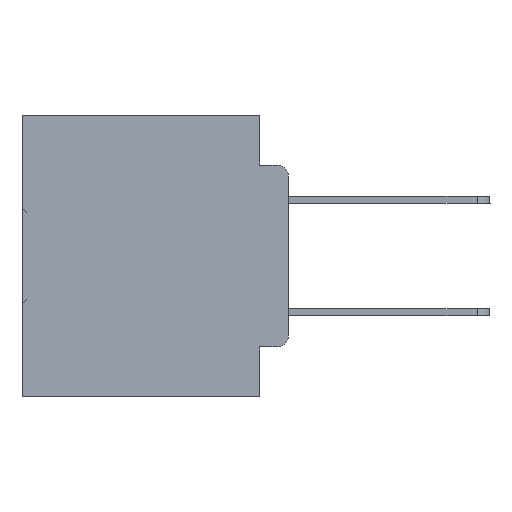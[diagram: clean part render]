
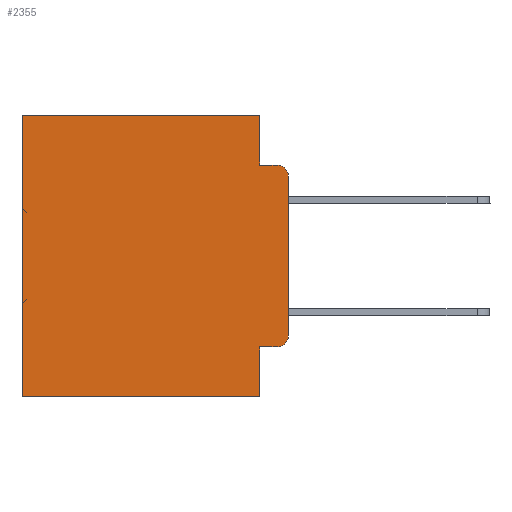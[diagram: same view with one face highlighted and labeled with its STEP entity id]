
A CAD part, left-side view. The second image highlights one B-rep face of the part: STEP entity #2355.
In plain terms, the highlighted planar face has unit normal (-1, 0, 0).
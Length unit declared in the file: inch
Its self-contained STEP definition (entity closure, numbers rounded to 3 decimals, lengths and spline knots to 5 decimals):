
#409 = VERTEX_POINT ( 'NONE', #15156 ) ;
#1267 = ORIENTED_EDGE ( 'NONE', *, *, #14678, .T. ) ;
#1294 = CARTESIAN_POINT ( 'NONE',  ( 0.298, 0.051, -0.0885 ) ) ;
#1667 = ORIENTED_EDGE ( 'NONE', *, *, #29807, .F. ) ;
#1814 = EDGE_CURVE ( 'NONE', #10155, #35746, #15122, .T. ) ;
#1840 = VECTOR ( 'NONE', #26566, 39.37008 ) ;
#2355 = ADVANCED_FACE ( 'NONE', ( #33717 ), #38267, .F. ) ;
#2360 = LINE ( 'NONE', #2878, #10711 ) ;
#2878 = CARTESIAN_POINT ( 'NONE',  ( 0.298, 0.051, 0. ) ) ;
#3962 = CARTESIAN_POINT ( 'NONE',  ( 0.298, 0.051, -0.5 ) ) ;
#5073 = LINE ( 'NONE', #1294, #34888 ) ;
#5926 = EDGE_CURVE ( 'NONE', #10482, #409, #16691, .T. ) ;
#6060 = DIRECTION ( 'NONE',  ( -1., 0., 0. ) ) ;
#6926 = CARTESIAN_POINT ( 'NONE',  ( 0.298, 0.051, 0. ) ) ;
#7176 = DIRECTION ( 'NONE',  ( 0., 1., 0. ) ) ;
#7782 = VECTOR ( 'NONE', #22080, 39.37008 ) ;
#8081 = VERTEX_POINT ( 'NONE', #37668 ) ;
#8518 = DIRECTION ( 'NONE',  ( 0., 0., -1. ) ) ;
#9224 = LINE ( 'NONE', #31961, #32115 ) ;
#9331 = CARTESIAN_POINT ( 'NONE',  ( 0.298, 0.051, -0.4115 ) ) ;
#10097 = DIRECTION ( 'NONE',  ( 0., -1., 0. ) ) ;
#10155 = VERTEX_POINT ( 'NONE', #32264 ) ;
#10190 = ORIENTED_EDGE ( 'NONE', *, *, #11402, .T. ) ;
#10482 = VERTEX_POINT ( 'NONE', #3962 ) ;
#10608 = LINE ( 'NONE', #25214, #7782 ) ;
#10711 = VECTOR ( 'NONE', #11688, 39.37008 ) ;
#11402 = EDGE_CURVE ( 'NONE', #12459, #8081, #35213, .T. ) ;
#11407 = VECTOR ( 'NONE', #7176, 39.37008 ) ;
#11688 = DIRECTION ( 'NONE',  ( 0., 0., -1. ) ) ;
#12317 = VECTOR ( 'NONE', #25186, 39.37008 ) ;
#12459 = VERTEX_POINT ( 'NONE', #6926 ) ;
#13038 = CARTESIAN_POINT ( 'NONE',  ( 0.298, 0., 0. ) ) ;
#13547 = CARTESIAN_POINT ( 'NONE',  ( 0.298, 0.051, -0.4115 ) ) ;
#13604 = ORIENTED_EDGE ( 'NONE', *, *, #34764, .F. ) ;
#13628 = CARTESIAN_POINT ( 'NONE',  ( 0.298, 0., -0.3915 ) ) ;
#14208 = DIRECTION ( 'NONE',  ( 0., 0., -1. ) ) ;
#14663 = ORIENTED_EDGE ( 'NONE', *, *, #37458, .T. ) ;
#14678 = EDGE_CURVE ( 'NONE', #8081, #409, #20279, .T. ) ;
#15054 = EDGE_LOOP ( 'NONE', ( #27919, #23209, #1667, #31357, #10190, #1267, #36738, #13604, #15475, #14663 ) ) ;
#15072 = VERTEX_POINT ( 'NONE', #13628 ) ;
#15122 = CIRCLE ( 'NONE', #37817, 0.02 ) ;
#15156 = CARTESIAN_POINT ( 'NONE',  ( 0.298, 0.473, -0.5 ) ) ;
#15475 = ORIENTED_EDGE ( 'NONE', *, *, #24546, .T. ) ;
#16691 = LINE ( 'NONE', #32827, #1840 ) ;
#17784 = CARTESIAN_POINT ( 'NONE',  ( 0.298, 0., 0. ) ) ;
#18313 = CARTESIAN_POINT ( 'NONE',  ( 0.298, 0.051, -0.0885 ) ) ;
#18534 = EDGE_CURVE ( 'NONE', #12459, #27743, #10608, .T. ) ;
#19207 = CARTESIAN_POINT ( 'NONE',  ( 0.298, 0.473, 0. ) ) ;
#19269 = EDGE_CURVE ( 'NONE', #10155, #15072, #9224, .T. ) ;
#19584 = DIRECTION ( 'NONE',  ( 0., 0., -1. ) ) ;
#20279 = LINE ( 'NONE', #19207, #12317 ) ;
#20367 = AXIS2_PLACEMENT_3D ( 'NONE', #17784, #23543, #8518 ) ;
#21932 = VECTOR ( 'NONE', #37300, 39.37008 ) ;
#22080 = DIRECTION ( 'NONE',  ( 0., 0., -1. ) ) ;
#23209 = ORIENTED_EDGE ( 'NONE', *, *, #1814, .T. ) ;
#23543 = DIRECTION ( 'NONE',  ( 1., 0., 0. ) ) ;
#23919 = CARTESIAN_POINT ( 'NONE',  ( 0.298, 0.02, -0.1085 ) ) ;
#24546 = EDGE_CURVE ( 'NONE', #29085, #25586, #29852, .T. ) ;
#25186 = DIRECTION ( 'NONE',  ( 0., 0., -1. ) ) ;
#25214 = CARTESIAN_POINT ( 'NONE',  ( 0.298, 0.051, 0. ) ) ;
#25586 = VERTEX_POINT ( 'NONE', #30829 ) ;
#26566 = DIRECTION ( 'NONE',  ( 0., 1., 0. ) ) ;
#27743 = VERTEX_POINT ( 'NONE', #18313 ) ;
#27919 = ORIENTED_EDGE ( 'NONE', *, *, #19269, .F. ) ;
#28329 = AXIS2_PLACEMENT_3D ( 'NONE', #37456, #37078, #19584 ) ;
#28807 = CARTESIAN_POINT ( 'NONE',  ( 0.298, 0.02, -0.0885 ) ) ;
#29085 = VERTEX_POINT ( 'NONE', #9331 ) ;
#29807 = EDGE_CURVE ( 'NONE', #27743, #35746, #5073, .T. ) ;
#29852 = LINE ( 'NONE', #13547, #21932 ) ;
#30829 = CARTESIAN_POINT ( 'NONE',  ( 0.298, 0.02, -0.4115 ) ) ;
#31357 = ORIENTED_EDGE ( 'NONE', *, *, #18534, .F. ) ;
#31961 = CARTESIAN_POINT ( 'NONE',  ( 0.298, 0., 0. ) ) ;
#32115 = VECTOR ( 'NONE', #14208, 39.37008 ) ;
#32264 = CARTESIAN_POINT ( 'NONE',  ( 0.298, 0., -0.1085 ) ) ;
#32827 = CARTESIAN_POINT ( 'NONE',  ( 0.298, 0., -0.5 ) ) ;
#33717 = FACE_OUTER_BOUND ( 'NONE', #15054, .T. ) ;
#34764 = EDGE_CURVE ( 'NONE', #29085, #10482, #2360, .T. ) ;
#34888 = VECTOR ( 'NONE', #10097, 39.37008 ) ;
#35213 = LINE ( 'NONE', #13038, #11407 ) ;
#35746 = VERTEX_POINT ( 'NONE', #28807 ) ;
#35923 = DIRECTION ( 'NONE',  ( 0., 0., -1. ) ) ;
#36738 = ORIENTED_EDGE ( 'NONE', *, *, #5926, .F. ) ;
#37078 = DIRECTION ( 'NONE',  ( -1., 0., 0. ) ) ;
#37300 = DIRECTION ( 'NONE',  ( 0., -1., 0. ) ) ;
#37456 = CARTESIAN_POINT ( 'NONE',  ( 0.298, 0.02, -0.3915 ) ) ;
#37458 = EDGE_CURVE ( 'NONE', #25586, #15072, #37559, .T. ) ;
#37559 = CIRCLE ( 'NONE', #28329, 0.02 ) ;
#37668 = CARTESIAN_POINT ( 'NONE',  ( 0.298, 0.473, 0. ) ) ;
#37817 = AXIS2_PLACEMENT_3D ( 'NONE', #23919, #6060, #35923 ) ;
#38267 = PLANE ( 'NONE',  #20367 ) ;
